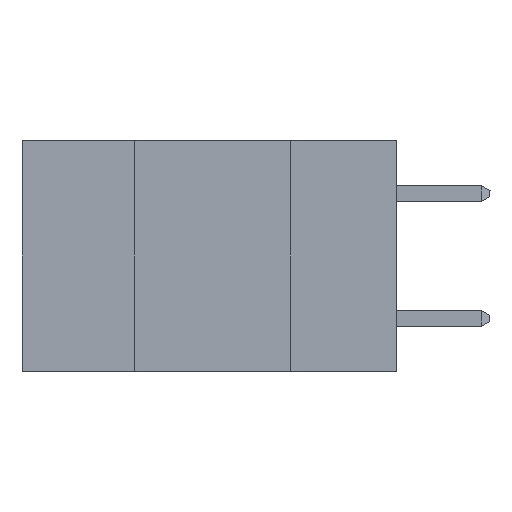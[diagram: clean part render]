
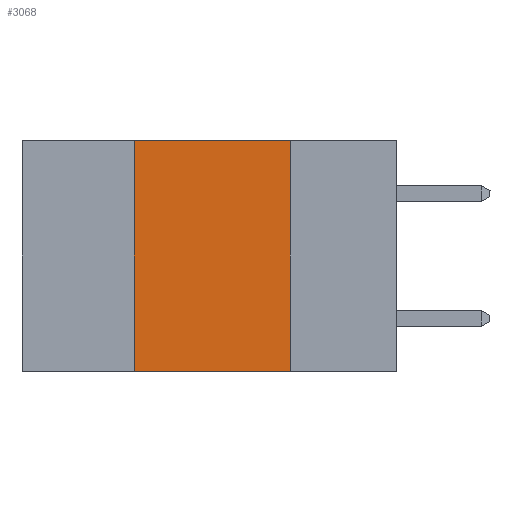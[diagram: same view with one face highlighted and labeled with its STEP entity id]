
A CAD part, left-side view. The second image highlights one B-rep face of the part: STEP entity #3068.
In plain terms, the highlighted planar face has unit normal (-1, 0, 0).
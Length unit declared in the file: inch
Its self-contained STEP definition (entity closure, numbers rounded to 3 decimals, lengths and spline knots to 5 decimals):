
#548 = CARTESIAN_POINT ( 'NONE',  ( 0., 0.17, 0. ) ) ;
#1467 = FACE_OUTER_BOUND ( 'NONE', #15060, .T. ) ;
#1651 = EDGE_CURVE ( 'NONE', #9438, #6234, #1993, .T. ) ;
#1993 = LINE ( 'NONE', #17912, #9221 ) ;
#2043 = DIRECTION ( 'NONE',  ( 0., 0., -1. ) ) ;
#2797 = CARTESIAN_POINT ( 'NONE',  ( 0., 0.42, 0. ) ) ;
#3068 = ADVANCED_FACE ( 'NONE', ( #1467 ), #9299, .F. ) ;
#3766 = VECTOR ( 'NONE', #12348, 39.37008 ) ;
#3965 = ORIENTED_EDGE ( 'NONE', *, *, #9865, .F. ) ;
#6008 = CARTESIAN_POINT ( 'NONE',  ( 0., 0.42, -0.37 ) ) ;
#6026 = VERTEX_POINT ( 'NONE', #11534 ) ;
#6234 = VERTEX_POINT ( 'NONE', #8312 ) ;
#7598 = LINE ( 'NONE', #17841, #3766 ) ;
#8312 = CARTESIAN_POINT ( 'NONE',  ( 0., 0.17, 0. ) ) ;
#8945 = EDGE_CURVE ( 'NONE', #15365, #6026, #7598, .T. ) ;
#9017 = DIRECTION ( 'NONE',  ( 0., -1., 0. ) ) ;
#9033 = LINE ( 'NONE', #548, #16061 ) ;
#9221 = VECTOR ( 'NONE', #9017, 39.37008 ) ;
#9222 = CARTESIAN_POINT ( 'NONE',  ( 0., 0.6, 0. ) ) ;
#9299 = PLANE ( 'NONE',  #14991 ) ;
#9438 = VERTEX_POINT ( 'NONE', #13304 ) ;
#9865 = EDGE_CURVE ( 'NONE', #15365, #9438, #10853, .T. ) ;
#10000 = DIRECTION ( 'NONE',  ( 0., 0., 1. ) ) ;
#10639 = ORIENTED_EDGE ( 'NONE', *, *, #1651, .F. ) ;
#10853 = LINE ( 'NONE', #2797, #17829 ) ;
#11534 = CARTESIAN_POINT ( 'NONE',  ( 0., 0.17, -0.37 ) ) ;
#11792 = EDGE_CURVE ( 'NONE', #6234, #6026, #9033, .T. ) ;
#12348 = DIRECTION ( 'NONE',  ( 0., -1., 0. ) ) ;
#13304 = CARTESIAN_POINT ( 'NONE',  ( 0., 0.42, 0. ) ) ;
#13309 = ORIENTED_EDGE ( 'NONE', *, *, #8945, .T. ) ;
#13525 = ORIENTED_EDGE ( 'NONE', *, *, #11792, .F. ) ;
#14779 = DIRECTION ( 'NONE',  ( 0., 0., -1. ) ) ;
#14830 = DIRECTION ( 'NONE',  ( 1., 0., 0. ) ) ;
#14991 = AXIS2_PLACEMENT_3D ( 'NONE', #9222, #14830, #14779 ) ;
#15060 = EDGE_LOOP ( 'NONE', ( #13525, #10639, #3965, #13309 ) ) ;
#15365 = VERTEX_POINT ( 'NONE', #6008 ) ;
#16061 = VECTOR ( 'NONE', #2043, 39.37008 ) ;
#17829 = VECTOR ( 'NONE', #10000, 39.37008 ) ;
#17841 = CARTESIAN_POINT ( 'NONE',  ( 0., 0.6, -0.37 ) ) ;
#17912 = CARTESIAN_POINT ( 'NONE',  ( 0., 0.6, 0. ) ) ;
